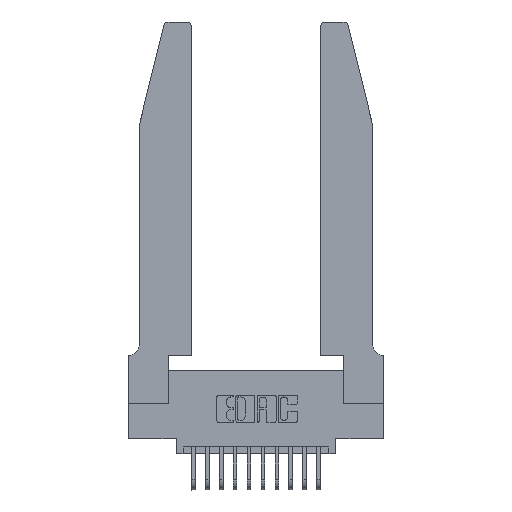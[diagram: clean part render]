
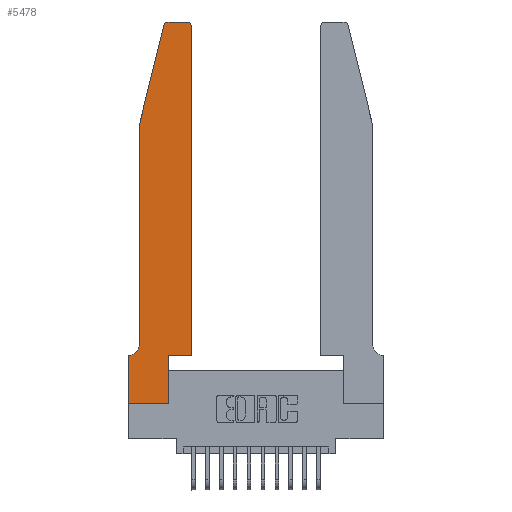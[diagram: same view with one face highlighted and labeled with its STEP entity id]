
A CAD part, top view. The second image highlights one B-rep face of the part: STEP entity #5478.
In plain terms, the highlighted planar face has unit normal (0, 0, 1).
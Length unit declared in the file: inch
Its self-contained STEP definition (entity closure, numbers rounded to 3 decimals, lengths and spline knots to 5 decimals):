
#100 = ORIENTED_EDGE ( 'NONE', *, *, #12018, .T. ) ;
#1288 = VERTEX_POINT ( 'NONE', #10784 ) ;
#1369 = ORIENTED_EDGE ( 'NONE', *, *, #3649, .T. ) ;
#1463 = CARTESIAN_POINT ( 'NONE',  ( 0.0755, 2., 0.37 ) ) ;
#1528 = VERTEX_POINT ( 'NONE', #4153 ) ;
#1637 = CARTESIAN_POINT ( 'NONE',  ( 0.2865, 0.35, 0.37 ) ) ;
#1824 = CARTESIAN_POINT ( 'NONE',  ( 0., 0., 0.37 ) ) ;
#2224 = VERTEX_POINT ( 'NONE', #10580 ) ;
#2614 = ORIENTED_EDGE ( 'NONE', *, *, #10391, .T. ) ;
#2687 = DIRECTION ( 'NONE',  ( -1., 0., 0. ) ) ;
#2768 = CIRCLE ( 'NONE', #7280, 0.03 ) ;
#2781 = LINE ( 'NONE', #12644, #6360 ) ;
#2791 = DIRECTION ( 'NONE',  ( -0.239, -0.971, 0. ) ) ;
#2804 = ORIENTED_EDGE ( 'NONE', *, *, #7770, .T. ) ;
#2930 = CARTESIAN_POINT ( 'NONE',  ( 0.284, 2.72, 0.37 ) ) ;
#2953 = CARTESIAN_POINT ( 'NONE',  ( 0.0055, 0.42, 0.37 ) ) ;
#3093 = PLANE ( 'NONE',  #15757 ) ;
#3174 = EDGE_CURVE ( 'NONE', #6466, #1288, #9918, .T. ) ;
#3208 = EDGE_CURVE ( 'NONE', #12365, #5019, #12894, .T. ) ;
#3454 = DIRECTION ( 'NONE',  ( 0., 1., 0. ) ) ;
#3649 = EDGE_CURVE ( 'NONE', #9063, #10953, #16101, .T. ) ;
#3847 = ORIENTED_EDGE ( 'NONE', *, *, #3927, .T. ) ;
#3927 = EDGE_CURVE ( 'NONE', #1288, #12365, #15136, .T. ) ;
#3944 = DIRECTION ( 'NONE',  ( 1., 0., 0. ) ) ;
#4092 = EDGE_CURVE ( 'NONE', #6735, #4482, #2781, .T. ) ;
#4153 = CARTESIAN_POINT ( 'NONE',  ( 0.2865, 0.35, 0.37 ) ) ;
#4302 = DIRECTION ( 'NONE',  ( 1., 0., 0. ) ) ;
#4322 = DIRECTION ( 'NONE',  ( -1., 0., 0. ) ) ;
#4417 = EDGE_CURVE ( 'NONE', #5019, #1528, #15122, .T. ) ;
#4464 = DIRECTION ( 'NONE',  ( 0., 0., 1. ) ) ;
#4482 = VERTEX_POINT ( 'NONE', #4695 ) ;
#4695 = CARTESIAN_POINT ( 'NONE',  ( 0.4505, 2.72, 0.37 ) ) ;
#4817 = EDGE_LOOP ( 'NONE', ( #100, #11304, #2804, #1369, #13631, #12265, #3847, #11299, #7209, #2614, #11531, #13478 ) ) ;
#4892 = CIRCLE ( 'NONE', #10516, 0.03 ) ;
#4926 = VECTOR ( 'NONE', #5877, 39.37008 ) ;
#5019 = VERTEX_POINT ( 'NONE', #16438 ) ;
#5033 = LINE ( 'NONE', #1463, #11202 ) ;
#5343 = EDGE_CURVE ( 'NONE', #2224, #13123, #2768, .T. ) ;
#5478 = ADVANCED_FACE ( 'NONE', ( #11271 ), #3093, .T. ) ;
#5560 = DIRECTION ( 'NONE',  ( -1., 0., 0. ) ) ;
#5667 = EDGE_CURVE ( 'NONE', #4482, #8575, #4892, .T. ) ;
#5877 = DIRECTION ( 'NONE',  ( 0., -1., 0. ) ) ;
#6028 = CARTESIAN_POINT ( 'NONE',  ( 0., 0., 0.37 ) ) ;
#6319 = LINE ( 'NONE', #9350, #9438 ) ;
#6360 = VECTOR ( 'NONE', #3454, 39.37008 ) ;
#6466 = VERTEX_POINT ( 'NONE', #14294 ) ;
#6534 = CARTESIAN_POINT ( 'NONE',  ( 0.4205, 2.75, 0.37 ) ) ;
#6644 = CARTESIAN_POINT ( 'NONE',  ( 0.25487, 2.72718, 0.37 ) ) ;
#6735 = VERTEX_POINT ( 'NONE', #9893 ) ;
#6767 = VECTOR ( 'NONE', #3944, 39.37008 ) ;
#6807 = VECTOR ( 'NONE', #5560, 39.37008 ) ;
#6920 = CIRCLE ( 'NONE', #10597, 0.07 ) ;
#7209 = ORIENTED_EDGE ( 'NONE', *, *, #4417, .T. ) ;
#7280 = AXIS2_PLACEMENT_3D ( 'NONE', #2930, #12144, #4302 ) ;
#7559 = DIRECTION ( 'NONE',  ( 0., 0., 1. ) ) ;
#7770 = EDGE_CURVE ( 'NONE', #13123, #9063, #5033, .T. ) ;
#8575 = VERTEX_POINT ( 'NONE', #6534 ) ;
#9063 = VERTEX_POINT ( 'NONE', #14010 ) ;
#9201 = DIRECTION ( 'NONE',  ( 0., -1., 0. ) ) ;
#9350 = CARTESIAN_POINT ( 'NONE',  ( 0.2605, 2.75, 0.37 ) ) ;
#9438 = VECTOR ( 'NONE', #2687, 39.37008 ) ;
#9618 = CARTESIAN_POINT ( 'NONE',  ( 0., 0., 0.37 ) ) ;
#9689 = DIRECTION ( 'NONE',  ( 0., 1., 0. ) ) ;
#9893 = CARTESIAN_POINT ( 'NONE',  ( 0.4505, 0.35, 0.37 ) ) ;
#9918 = LINE ( 'NONE', #13322, #6807 ) ;
#10391 = EDGE_CURVE ( 'NONE', #1528, #6735, #15693, .T. ) ;
#10516 = AXIS2_PLACEMENT_3D ( 'NONE', #15137, #7559, #16413 ) ;
#10580 = CARTESIAN_POINT ( 'NONE',  ( 0.284, 2.75, 0.37 ) ) ;
#10597 = AXIS2_PLACEMENT_3D ( 'NONE', #2953, #12167, #4322 ) ;
#10784 = CARTESIAN_POINT ( 'NONE',  ( 0., 0.35, 0.37 ) ) ;
#10953 = VERTEX_POINT ( 'NONE', #12112 ) ;
#11202 = VECTOR ( 'NONE', #2791, 39.37008 ) ;
#11271 = FACE_OUTER_BOUND ( 'NONE', #4817, .T. ) ;
#11299 = ORIENTED_EDGE ( 'NONE', *, *, #3208, .T. ) ;
#11304 = ORIENTED_EDGE ( 'NONE', *, *, #5343, .T. ) ;
#11531 = ORIENTED_EDGE ( 'NONE', *, *, #4092, .T. ) ;
#11868 = VECTOR ( 'NONE', #9689, 39.37008 ) ;
#12018 = EDGE_CURVE ( 'NONE', #8575, #2224, #6319, .T. ) ;
#12110 = DIRECTION ( 'NONE',  ( 1., 0., 0. ) ) ;
#12112 = CARTESIAN_POINT ( 'NONE',  ( 0.0755, 0.42, 0.37 ) ) ;
#12144 = DIRECTION ( 'NONE',  ( 0., 0., 1. ) ) ;
#12167 = DIRECTION ( 'NONE',  ( 0., 0., -1. ) ) ;
#12265 = ORIENTED_EDGE ( 'NONE', *, *, #3174, .T. ) ;
#12308 = CARTESIAN_POINT ( 'NONE',  ( 0., 0.35, 0.37 ) ) ;
#12365 = VERTEX_POINT ( 'NONE', #6028 ) ;
#12644 = CARTESIAN_POINT ( 'NONE',  ( 0.4505, 0.35, 0.37 ) ) ;
#12649 = EDGE_CURVE ( 'NONE', #10953, #6466, #6920, .T. ) ;
#12894 = LINE ( 'NONE', #9618, #15729 ) ;
#13114 = CARTESIAN_POINT ( 'NONE',  ( 0.4505, 0.35, 0.37 ) ) ;
#13123 = VERTEX_POINT ( 'NONE', #6644 ) ;
#13322 = CARTESIAN_POINT ( 'NONE',  ( 0.0755, 0.35, 0.37 ) ) ;
#13478 = ORIENTED_EDGE ( 'NONE', *, *, #5667, .T. ) ;
#13564 = DIRECTION ( 'NONE',  ( 1., 0., 0. ) ) ;
#13631 = ORIENTED_EDGE ( 'NONE', *, *, #12649, .T. ) ;
#14010 = CARTESIAN_POINT ( 'NONE',  ( 0.0755, 2., 0.37 ) ) ;
#14294 = CARTESIAN_POINT ( 'NONE',  ( 0.0055, 0.35, 0.37 ) ) ;
#14417 = VECTOR ( 'NONE', #9201, 39.37008 ) ;
#15122 = LINE ( 'NONE', #1637, #11868 ) ;
#15136 = LINE ( 'NONE', #1824, #4926 ) ;
#15137 = CARTESIAN_POINT ( 'NONE',  ( 0.4205, 2.72, 0.37 ) ) ;
#15419 = CARTESIAN_POINT ( 'NONE',  ( 0.0755, 2., 0.37 ) ) ;
#15693 = LINE ( 'NONE', #13114, #6767 ) ;
#15729 = VECTOR ( 'NONE', #12110, 39.37008 ) ;
#15757 = AXIS2_PLACEMENT_3D ( 'NONE', #12308, #4464, #13564 ) ;
#16101 = LINE ( 'NONE', #15419, #14417 ) ;
#16413 = DIRECTION ( 'NONE',  ( 1., 0., 0. ) ) ;
#16438 = CARTESIAN_POINT ( 'NONE',  ( 0.2865, 0., 0.37 ) ) ;
